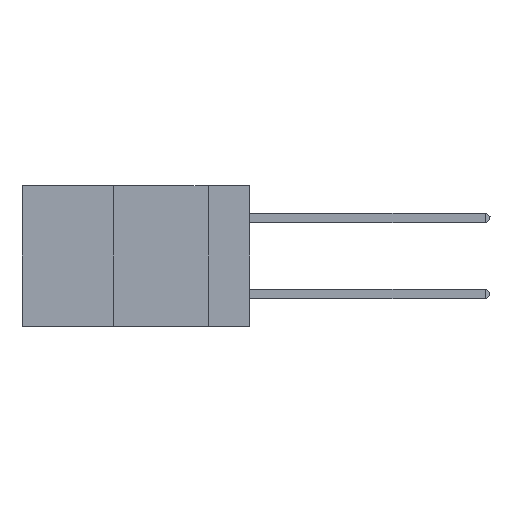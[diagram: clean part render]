
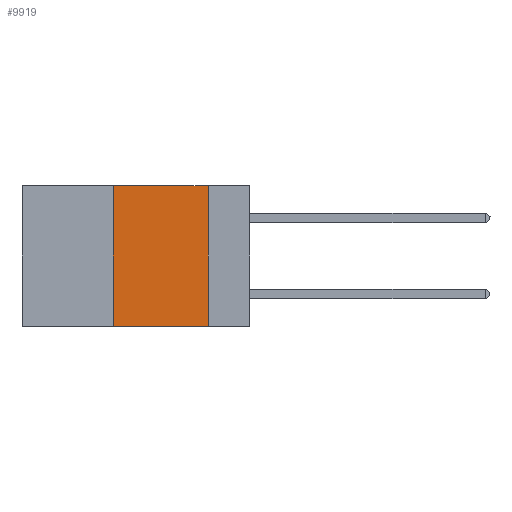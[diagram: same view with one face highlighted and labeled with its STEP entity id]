
A CAD part, left-side view. The second image highlights one B-rep face of the part: STEP entity #9919.
In plain terms, the highlighted planar face has unit normal (-1, 0, 0).
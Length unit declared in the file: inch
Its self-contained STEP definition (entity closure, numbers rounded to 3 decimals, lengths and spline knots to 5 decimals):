
#286 = CARTESIAN_POINT ( 'NONE',  ( 0., 0.36, -0.37 ) ) ;
#1152 = DIRECTION ( 'NONE',  ( 0., 0., 1. ) ) ;
#1224 = PLANE ( 'NONE',  #1665 ) ;
#1603 = LINE ( 'NONE', #3389, #14110 ) ;
#1665 = AXIS2_PLACEMENT_3D ( 'NONE', #6940, #11275, #19025 ) ;
#2040 = LINE ( 'NONE', #19189, #7835 ) ;
#2581 = ORIENTED_EDGE ( 'NONE', *, *, #2962, .F. ) ;
#2744 = VERTEX_POINT ( 'NONE', #286 ) ;
#2962 = EDGE_CURVE ( 'NONE', #20558, #11665, #9281, .T. ) ;
#3389 = CARTESIAN_POINT ( 'NONE',  ( 0., 0.6, -0.37 ) ) ;
#3630 = CARTESIAN_POINT ( 'NONE',  ( 0., 0.11, 0. ) ) ;
#5359 = EDGE_CURVE ( 'NONE', #2744, #24715, #1603, .T. ) ;
#5426 = DIRECTION ( 'NONE',  ( 0., -1., 0. ) ) ;
#6940 = CARTESIAN_POINT ( 'NONE',  ( 0., 0.6, 0. ) ) ;
#7835 = VECTOR ( 'NONE', #9778, 39.37008 ) ;
#9019 = DIRECTION ( 'NONE',  ( 0., -1., 0. ) ) ;
#9086 = CARTESIAN_POINT ( 'NONE',  ( 0., 0.11, -0.37 ) ) ;
#9103 = FACE_OUTER_BOUND ( 'NONE', #14394, .T. ) ;
#9281 = LINE ( 'NONE', #9527, #10761 ) ;
#9527 = CARTESIAN_POINT ( 'NONE',  ( 0., 0.6, 0. ) ) ;
#9778 = DIRECTION ( 'NONE',  ( 0., 0., -1. ) ) ;
#9919 = ADVANCED_FACE ( 'NONE', ( #9103 ), #1224, .F. ) ;
#10694 = CARTESIAN_POINT ( 'NONE',  ( 0., 0.36, 0. ) ) ;
#10761 = VECTOR ( 'NONE', #9019, 39.37008 ) ;
#11065 = ORIENTED_EDGE ( 'NONE', *, *, #5359, .T. ) ;
#11275 = DIRECTION ( 'NONE',  ( 1., 0., 0. ) ) ;
#11665 = VERTEX_POINT ( 'NONE', #3630 ) ;
#12036 = VECTOR ( 'NONE', #1152, 39.37008 ) ;
#14110 = VECTOR ( 'NONE', #5426, 39.37008 ) ;
#14394 = EDGE_LOOP ( 'NONE', ( #20577, #2581, #24790, #11065 ) ) ;
#17012 = CARTESIAN_POINT ( 'NONE',  ( 0., 0.36, 0. ) ) ;
#18577 = LINE ( 'NONE', #10694, #12036 ) ;
#18972 = EDGE_CURVE ( 'NONE', #2744, #20558, #18577, .T. ) ;
#19025 = DIRECTION ( 'NONE',  ( 0., 0., -1. ) ) ;
#19189 = CARTESIAN_POINT ( 'NONE',  ( 0., 0.11, 0. ) ) ;
#20558 = VERTEX_POINT ( 'NONE', #17012 ) ;
#20577 = ORIENTED_EDGE ( 'NONE', *, *, #23872, .F. ) ;
#23872 = EDGE_CURVE ( 'NONE', #11665, #24715, #2040, .T. ) ;
#24715 = VERTEX_POINT ( 'NONE', #9086 ) ;
#24790 = ORIENTED_EDGE ( 'NONE', *, *, #18972, .F. ) ;
